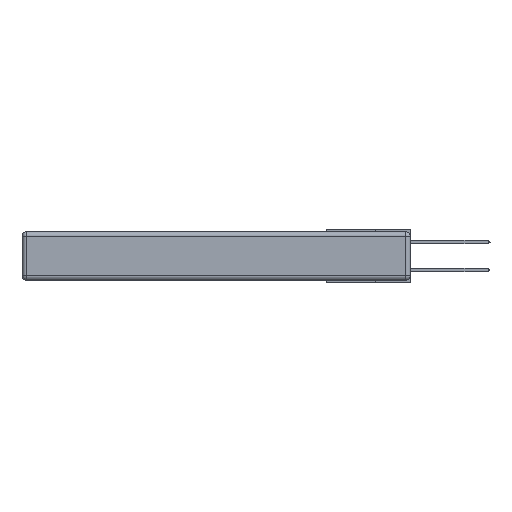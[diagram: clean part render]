
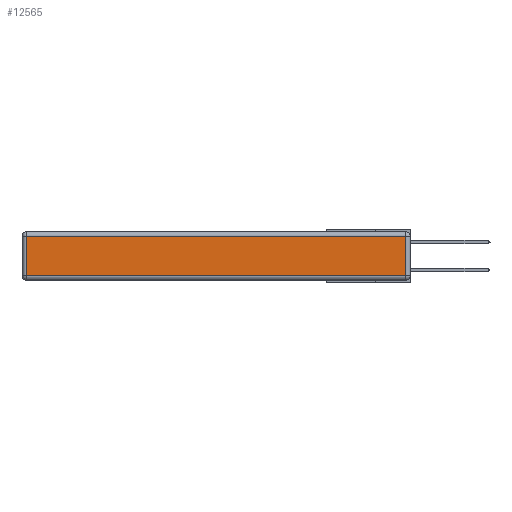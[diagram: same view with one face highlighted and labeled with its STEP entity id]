
A CAD part, left-side view. The second image highlights one B-rep face of the part: STEP entity #12565.
In plain terms, the highlighted planar face has unit normal (-1, 0, 0).
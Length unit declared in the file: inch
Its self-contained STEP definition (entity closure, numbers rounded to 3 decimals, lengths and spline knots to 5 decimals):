
#227 = EDGE_LOOP ( 'NONE', ( #4381, #15724, #11140, #1822 ) ) ;
#374 = CARTESIAN_POINT ( 'NONE',  ( 0., 0.03, -0.03 ) ) ;
#710 = DIRECTION ( 'NONE',  ( 0., 1., 0. ) ) ;
#1822 = ORIENTED_EDGE ( 'NONE', *, *, #7230, .T. ) ;
#2033 = CARTESIAN_POINT ( 'NONE',  ( 0., 0., -0.343 ) ) ;
#2054 = DIRECTION ( 'NONE',  ( 0., 0., -1. ) ) ;
#2644 = VERTEX_POINT ( 'NONE', #10988 ) ;
#3287 = PLANE ( 'NONE',  #13374 ) ;
#4008 = VECTOR ( 'NONE', #2054, 39.37008 ) ;
#4381 = ORIENTED_EDGE ( 'NONE', *, *, #13146, .T. ) ;
#4807 = CARTESIAN_POINT ( 'NONE',  ( 0., 2.72, -0.343 ) ) ;
#4967 = CARTESIAN_POINT ( 'NONE',  ( 0., 0., -0.313 ) ) ;
#5444 = VERTEX_POINT ( 'NONE', #9912 ) ;
#5929 = DIRECTION ( 'NONE',  ( -1., 0., 0. ) ) ;
#6175 = VECTOR ( 'NONE', #710, 39.37008 ) ;
#6189 = VECTOR ( 'NONE', #8858, 39.37008 ) ;
#7228 = DIRECTION ( 'NONE',  ( 0., 0., 1. ) ) ;
#7230 = EDGE_CURVE ( 'NONE', #5444, #8772, #8074, .T. ) ;
#7693 = VERTEX_POINT ( 'NONE', #374 ) ;
#8074 = LINE ( 'NONE', #4807, #4008 ) ;
#8707 = CARTESIAN_POINT ( 'NONE',  ( 0., 0.03, -0.343 ) ) ;
#8772 = VERTEX_POINT ( 'NONE', #14449 ) ;
#8858 = DIRECTION ( 'NONE',  ( 0., 0., 1. ) ) ;
#9253 = EDGE_CURVE ( 'NONE', #7693, #5444, #14811, .T. ) ;
#9619 = LINE ( 'NONE', #8707, #6189 ) ;
#9912 = CARTESIAN_POINT ( 'NONE',  ( 0., 2.72, -0.03 ) ) ;
#10262 = EDGE_CURVE ( 'NONE', #2644, #7693, #9619, .T. ) ;
#10730 = VECTOR ( 'NONE', #11449, 39.37008 ) ;
#10988 = CARTESIAN_POINT ( 'NONE',  ( 0., 0.03, -0.313 ) ) ;
#11140 = ORIENTED_EDGE ( 'NONE', *, *, #9253, .T. ) ;
#11449 = DIRECTION ( 'NONE',  ( 0., -1., 0. ) ) ;
#12565 = ADVANCED_FACE ( 'NONE', ( #13740 ), #3287, .T. ) ;
#13146 = EDGE_CURVE ( 'NONE', #8772, #2644, #14118, .T. ) ;
#13374 = AXIS2_PLACEMENT_3D ( 'NONE', #2033, #5929, #7228 ) ;
#13740 = FACE_OUTER_BOUND ( 'NONE', #227, .T. ) ;
#14118 = LINE ( 'NONE', #4967, #10730 ) ;
#14449 = CARTESIAN_POINT ( 'NONE',  ( 0., 2.72, -0.313 ) ) ;
#14760 = CARTESIAN_POINT ( 'NONE',  ( 0., 2.75, -0.03 ) ) ;
#14811 = LINE ( 'NONE', #14760, #6175 ) ;
#15724 = ORIENTED_EDGE ( 'NONE', *, *, #10262, .T. ) ;
